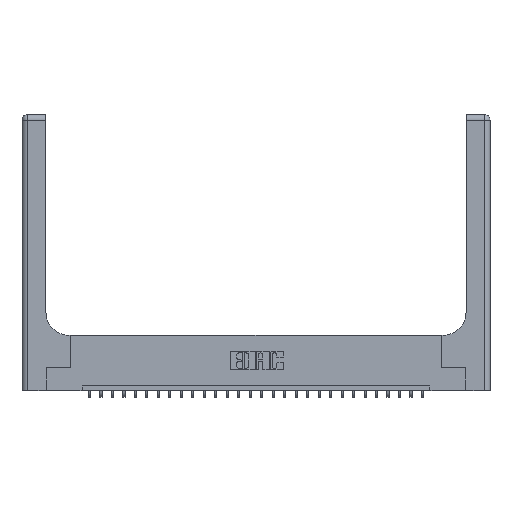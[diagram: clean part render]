
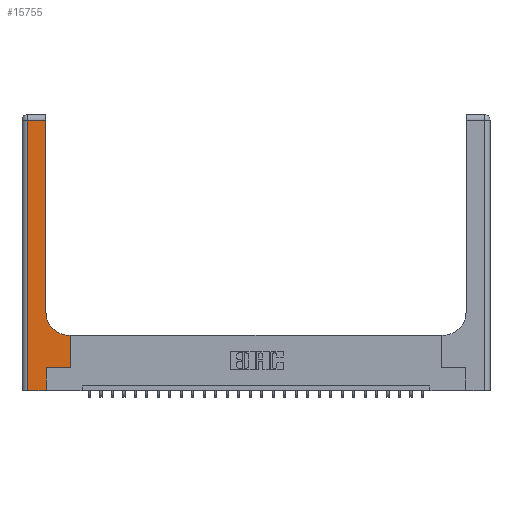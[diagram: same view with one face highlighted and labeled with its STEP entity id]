
A CAD part, top view. The second image highlights one B-rep face of the part: STEP entity #15755.
In plain terms, the highlighted planar face has unit normal (0, 0, 1).
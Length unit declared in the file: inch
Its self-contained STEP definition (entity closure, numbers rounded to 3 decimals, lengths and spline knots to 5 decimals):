
#402 = CARTESIAN_POINT ( 'NONE',  ( 0.51, 0.6, 0.37 ) ) ;
#918 = CARTESIAN_POINT ( 'NONE',  ( 0., 0., 0.37 ) ) ;
#1438 = DIRECTION ( 'NONE',  ( 1., 0., 0. ) ) ;
#1641 = DIRECTION ( 'NONE',  ( 0., 0., -1. ) ) ;
#1972 = FACE_OUTER_BOUND ( 'NONE', #7422, .T. ) ;
#2102 = DIRECTION ( 'NONE',  ( 0., 0., -1. ) ) ;
#2667 = VERTEX_POINT ( 'NONE', #18292 ) ;
#2687 = LINE ( 'NONE', #24842, #6968 ) ;
#2768 = VECTOR ( 'NONE', #1438, 39.37008 ) ;
#3081 = CARTESIAN_POINT ( 'NONE',  ( 0.26, 0.85, 0.37 ) ) ;
#3273 = DIRECTION ( 'NONE',  ( 0., -1., 0. ) ) ;
#3522 = CARTESIAN_POINT ( 'NONE',  ( 0.265, 0., 0.37 ) ) ;
#3972 = VERTEX_POINT ( 'NONE', #11362 ) ;
#4300 = EDGE_CURVE ( 'NONE', #7740, #24494, #20460, .T. ) ;
#4825 = CARTESIAN_POINT ( 'NONE',  ( 0.26, 3., 0.37 ) ) ;
#5299 = DIRECTION ( 'NONE',  ( 1., 0., 0. ) ) ;
#5310 = LINE ( 'NONE', #8997, #20463 ) ;
#5438 = CARTESIAN_POINT ( 'NONE',  ( 0.51, 0.85, 0.37 ) ) ;
#5505 = VERTEX_POINT ( 'NONE', #15936 ) ;
#6127 = EDGE_CURVE ( 'NONE', #11976, #12473, #21479, .T. ) ;
#6681 = DIRECTION ( 'NONE',  ( 0., 1., 0. ) ) ;
#6817 = LINE ( 'NONE', #918, #2768 ) ;
#6914 = CARTESIAN_POINT ( 'NONE',  ( 0.528, 0.25, 0.37 ) ) ;
#6947 = ORIENTED_EDGE ( 'NONE', *, *, #15223, .T. ) ;
#6968 = VECTOR ( 'NONE', #20631, 39.37008 ) ;
#7422 = EDGE_LOOP ( 'NONE', ( #8259, #16791, #16655, #19538, #21484, #10123, #6947, #13774, #21495 ) ) ;
#7740 = VERTEX_POINT ( 'NONE', #8368 ) ;
#7905 = DIRECTION ( 'NONE',  ( 1., 0., 0. ) ) ;
#8038 = CARTESIAN_POINT ( 'NONE',  ( 0.265, 0.25, 0.37 ) ) ;
#8259 = ORIENTED_EDGE ( 'NONE', *, *, #16126, .T. ) ;
#8368 = CARTESIAN_POINT ( 'NONE',  ( 0.528, 0.6, 0.37 ) ) ;
#8899 = LINE ( 'NONE', #4825, #18000 ) ;
#8997 = CARTESIAN_POINT ( 'NONE',  ( 0.528, 0.25, 0.37 ) ) ;
#9127 = VECTOR ( 'NONE', #11906, 39.37008 ) ;
#9553 = AXIS2_PLACEMENT_3D ( 'NONE', #5438, #1641, #5299 ) ;
#10123 = ORIENTED_EDGE ( 'NONE', *, *, #12795, .T. ) ;
#10310 = CARTESIAN_POINT ( 'NONE',  ( 0.265, 0., 0.37 ) ) ;
#10395 = VECTOR ( 'NONE', #7905, 39.37008 ) ;
#11362 = CARTESIAN_POINT ( 'NONE',  ( 0.06, 0., 0.37 ) ) ;
#11906 = DIRECTION ( 'NONE',  ( 0., 1., 0. ) ) ;
#11976 = VERTEX_POINT ( 'NONE', #10310 ) ;
#12473 = VERTEX_POINT ( 'NONE', #18643 ) ;
#12795 = EDGE_CURVE ( 'NONE', #12473, #22478, #21918, .T. ) ;
#13292 = DIRECTION ( 'NONE',  ( 0., 1., 0. ) ) ;
#13774 = ORIENTED_EDGE ( 'NONE', *, *, #4300, .T. ) ;
#13887 = DIRECTION ( 'NONE',  ( -1., 0., 0. ) ) ;
#14009 = CARTESIAN_POINT ( 'NONE',  ( 0., 3., 0.37 ) ) ;
#14185 = DIRECTION ( 'NONE',  ( -1., 0., 0. ) ) ;
#15223 = EDGE_CURVE ( 'NONE', #22478, #7740, #5310, .T. ) ;
#15593 = LINE ( 'NONE', #21490, #17574 ) ;
#15755 = ADVANCED_FACE ( 'NONE', ( #1972 ), #25829, .F. ) ;
#15889 = EDGE_CURVE ( 'NONE', #2667, #3972, #15593, .T. ) ;
#15936 = CARTESIAN_POINT ( 'NONE',  ( 0.26, 2.94, 0.37 ) ) ;
#16126 = EDGE_CURVE ( 'NONE', #18220, #5505, #8899, .T. ) ;
#16349 = VECTOR ( 'NONE', #14185, 39.37008 ) ;
#16655 = ORIENTED_EDGE ( 'NONE', *, *, #15889, .T. ) ;
#16791 = ORIENTED_EDGE ( 'NONE', *, *, #21819, .T. ) ;
#17574 = VECTOR ( 'NONE', #3273, 39.37008 ) ;
#18000 = VECTOR ( 'NONE', #6681, 39.37008 ) ;
#18122 = CARTESIAN_POINT ( 'NONE',  ( 0.26, 0.6, 0.37 ) ) ;
#18220 = VERTEX_POINT ( 'NONE', #3081 ) ;
#18292 = CARTESIAN_POINT ( 'NONE',  ( 0.06, 2.94, 0.37 ) ) ;
#18643 = CARTESIAN_POINT ( 'NONE',  ( 0.265, 0.25, 0.37 ) ) ;
#19538 = ORIENTED_EDGE ( 'NONE', *, *, #24667, .T. ) ;
#20460 = LINE ( 'NONE', #18122, #16349 ) ;
#20463 = VECTOR ( 'NONE', #13292, 39.37008 ) ;
#20631 = DIRECTION ( 'NONE',  ( -1., 0., 0. ) ) ;
#21233 = CIRCLE ( 'NONE', #9553, 0.25 ) ;
#21479 = LINE ( 'NONE', #3522, #9127 ) ;
#21484 = ORIENTED_EDGE ( 'NONE', *, *, #6127, .T. ) ;
#21490 = CARTESIAN_POINT ( 'NONE',  ( 0.06, 3., 0.37 ) ) ;
#21495 = ORIENTED_EDGE ( 'NONE', *, *, #23136, .T. ) ;
#21819 = EDGE_CURVE ( 'NONE', #5505, #2667, #2687, .T. ) ;
#21918 = LINE ( 'NONE', #8038, #10395 ) ;
#22478 = VERTEX_POINT ( 'NONE', #6914 ) ;
#23004 = AXIS2_PLACEMENT_3D ( 'NONE', #14009, #2102, #13887 ) ;
#23136 = EDGE_CURVE ( 'NONE', #24494, #18220, #21233, .T. ) ;
#24494 = VERTEX_POINT ( 'NONE', #402 ) ;
#24667 = EDGE_CURVE ( 'NONE', #3972, #11976, #6817, .T. ) ;
#24842 = CARTESIAN_POINT ( 'NONE',  ( 0., 2.94, 0.37 ) ) ;
#25829 = PLANE ( 'NONE',  #23004 ) ;
